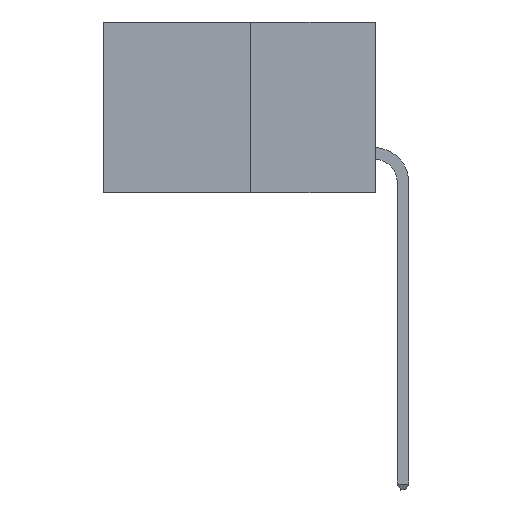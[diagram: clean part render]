
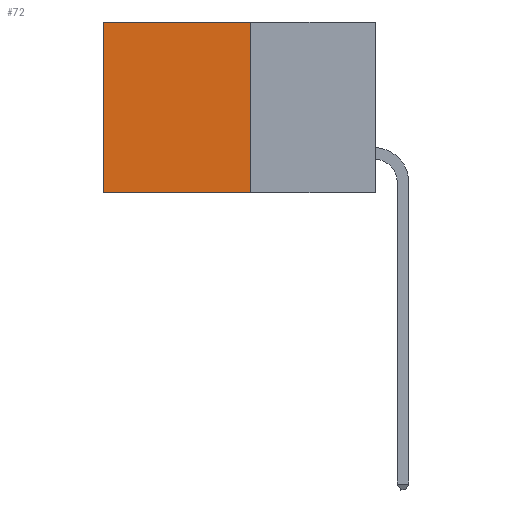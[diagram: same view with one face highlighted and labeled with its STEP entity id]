
A CAD part, left-side view. The second image highlights one B-rep face of the part: STEP entity #72.
In plain terms, the highlighted planar face has unit normal (-1, 0, 0).
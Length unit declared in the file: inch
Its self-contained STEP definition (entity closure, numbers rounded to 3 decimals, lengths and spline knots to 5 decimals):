
#72 = ADVANCED_FACE ( 'NONE', ( #21649 ), #2890, .F. ) ;
#325 = LINE ( 'NONE', #11321, #4999 ) ;
#1359 = ORIENTED_EDGE ( 'NONE', *, *, #16437, .F. ) ;
#2099 = CARTESIAN_POINT ( 'NONE',  ( 0.277, 0.27, -0.37 ) ) ;
#2890 = PLANE ( 'NONE',  #20523 ) ;
#3848 = DIRECTION ( 'NONE',  ( 0., 0., -1. ) ) ;
#3927 = CARTESIAN_POINT ( 'NONE',  ( 0.277, 0.27, 0. ) ) ;
#4080 = VERTEX_POINT ( 'NONE', #8311 ) ;
#4359 = DIRECTION ( 'NONE',  ( 0., 0., -1. ) ) ;
#4999 = VECTOR ( 'NONE', #4359, 39.37008 ) ;
#6218 = LINE ( 'NONE', #20566, #14916 ) ;
#6934 = LINE ( 'NONE', #2099, #11035 ) ;
#8311 = CARTESIAN_POINT ( 'NONE',  ( 0.277, 0.27, -0.37 ) ) ;
#8354 = LINE ( 'NONE', #14314, #22099 ) ;
#9132 = EDGE_CURVE ( 'NONE', #15544, #4080, #325, .T. ) ;
#9176 = DIRECTION ( 'NONE',  ( 0., 1., 0. ) ) ;
#11035 = VECTOR ( 'NONE', #12541, 39.37008 ) ;
#11321 = CARTESIAN_POINT ( 'NONE',  ( 0.277, 0.27, -0.37 ) ) ;
#12282 = ORIENTED_EDGE ( 'NONE', *, *, #9132, .F. ) ;
#12449 = EDGE_CURVE ( 'NONE', #15514, #14558, #6218, .T. ) ;
#12541 = DIRECTION ( 'NONE',  ( 0., 1., 0. ) ) ;
#13558 = CARTESIAN_POINT ( 'NONE',  ( 0.277, 0.59, -0.37 ) ) ;
#14314 = CARTESIAN_POINT ( 'NONE',  ( 0.277, 0.27, 0. ) ) ;
#14558 = VERTEX_POINT ( 'NONE', #13558 ) ;
#14916 = VECTOR ( 'NONE', #22232, 39.37008 ) ;
#15514 = VERTEX_POINT ( 'NONE', #21142 ) ;
#15544 = VERTEX_POINT ( 'NONE', #3927 ) ;
#15855 = EDGE_CURVE ( 'NONE', #15544, #15514, #8354, .T. ) ;
#16030 = DIRECTION ( 'NONE',  ( 1., 0., 0. ) ) ;
#16437 = EDGE_CURVE ( 'NONE', #4080, #14558, #6934, .T. ) ;
#16711 = CARTESIAN_POINT ( 'NONE',  ( 0.277, 0.27, -0.37 ) ) ;
#17079 = EDGE_LOOP ( 'NONE', ( #19040, #1359, #12282, #22041 ) ) ;
#19040 = ORIENTED_EDGE ( 'NONE', *, *, #12449, .T. ) ;
#20523 = AXIS2_PLACEMENT_3D ( 'NONE', #16711, #16030, #3848 ) ;
#20566 = CARTESIAN_POINT ( 'NONE',  ( 0.277, 0.59, -0.37 ) ) ;
#21142 = CARTESIAN_POINT ( 'NONE',  ( 0.277, 0.59, 0. ) ) ;
#21649 = FACE_OUTER_BOUND ( 'NONE', #17079, .T. ) ;
#22041 = ORIENTED_EDGE ( 'NONE', *, *, #15855, .T. ) ;
#22099 = VECTOR ( 'NONE', #9176, 39.37008 ) ;
#22232 = DIRECTION ( 'NONE',  ( 0., 0., -1. ) ) ;
